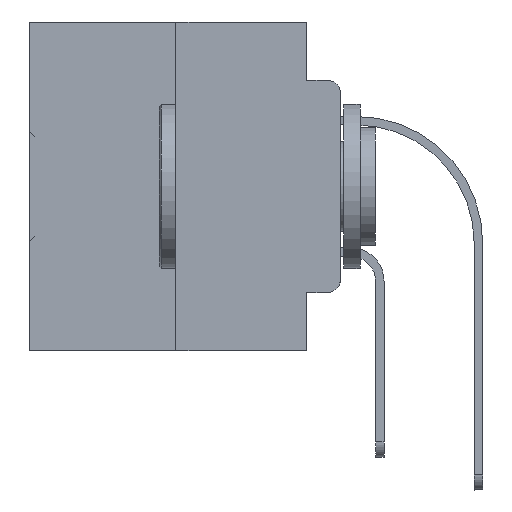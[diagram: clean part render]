
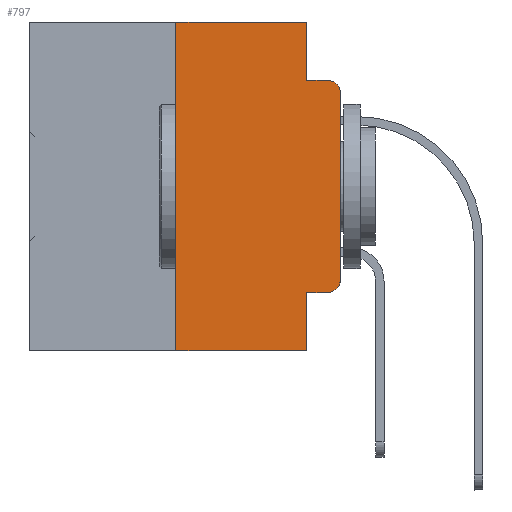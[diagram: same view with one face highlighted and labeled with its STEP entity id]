
A CAD part, left-side view. The second image highlights one B-rep face of the part: STEP entity #797.
In plain terms, the highlighted planar face has unit normal (-1, 0, 0).
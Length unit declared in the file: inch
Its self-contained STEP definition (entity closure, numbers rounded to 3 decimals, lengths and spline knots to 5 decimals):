
#170 = ORIENTED_EDGE ( 'NONE', *, *, #8537, .T. ) ;
#797 = ADVANCED_FACE ( 'NONE', ( #30992 ), #1287, .F. ) ;
#883 = CARTESIAN_POINT ( 'NONE',  ( 0., 0.473, 0. ) ) ;
#1096 = ORIENTED_EDGE ( 'NONE', *, *, #7318, .F. ) ;
#1287 = PLANE ( 'NONE',  #10939 ) ;
#1345 = VERTEX_POINT ( 'NONE', #14039 ) ;
#3352 = CARTESIAN_POINT ( 'NONE',  ( 0., 0.473, -0.5 ) ) ;
#3645 = LINE ( 'NONE', #18437, #16401 ) ;
#3656 = CARTESIAN_POINT ( 'NONE',  ( 0., 0.051, -0.0885 ) ) ;
#4393 = DIRECTION ( 'NONE',  ( 1., 0., 0. ) ) ;
#6863 = CARTESIAN_POINT ( 'NONE',  ( 0., 0., -0.1085 ) ) ;
#6879 = ORIENTED_EDGE ( 'NONE', *, *, #21582, .T. ) ;
#7318 = EDGE_CURVE ( 'NONE', #8456, #8293, #36587, .T. ) ;
#8228 = VECTOR ( 'NONE', #30574, 39.37008 ) ;
#8293 = VERTEX_POINT ( 'NONE', #17442 ) ;
#8456 = VERTEX_POINT ( 'NONE', #23482 ) ;
#8537 = EDGE_CURVE ( 'NONE', #38240, #11302, #30975, .T. ) ;
#8684 = EDGE_CURVE ( 'NONE', #8293, #34382, #36230, .T. ) ;
#8834 = ORIENTED_EDGE ( 'NONE', *, *, #22237, .F. ) ;
#8986 = CARTESIAN_POINT ( 'NONE',  ( 0., 0.02, -0.1085 ) ) ;
#9267 = EDGE_CURVE ( 'NONE', #34382, #1345, #3645, .T. ) ;
#9439 = ORIENTED_EDGE ( 'NONE', *, *, #9267, .F. ) ;
#9651 = CARTESIAN_POINT ( 'NONE',  ( 0., 0.051, 0. ) ) ;
#9960 = VERTEX_POINT ( 'NONE', #31731 ) ;
#10237 = DIRECTION ( 'NONE',  ( 0., 0., -1. ) ) ;
#10436 = AXIS2_PLACEMENT_3D ( 'NONE', #34102, #12779, #10237 ) ;
#10939 = AXIS2_PLACEMENT_3D ( 'NONE', #31196, #4393, #28299 ) ;
#11302 = VERTEX_POINT ( 'NONE', #36538 ) ;
#11423 = DIRECTION ( 'NONE',  ( 0., 0., 1. ) ) ;
#12779 = DIRECTION ( 'NONE',  ( -1., 0., 0. ) ) ;
#12907 = CIRCLE ( 'NONE', #10436, 0.02 ) ;
#13124 = CARTESIAN_POINT ( 'NONE',  ( 0., 0., 0. ) ) ;
#13659 = ORIENTED_EDGE ( 'NONE', *, *, #18242, .T. ) ;
#13963 = CARTESIAN_POINT ( 'NONE',  ( 0., 0.25, 0. ) ) ;
#14039 = CARTESIAN_POINT ( 'NONE',  ( 0., 0.02, -0.0885 ) ) ;
#15121 = VECTOR ( 'NONE', #21505, 39.37008 ) ;
#15213 = DIRECTION ( 'NONE',  ( -1., 0., 0. ) ) ;
#16401 = VECTOR ( 'NONE', #27344, 39.37008 ) ;
#16429 = ORIENTED_EDGE ( 'NONE', *, *, #33892, .F. ) ;
#16442 = LINE ( 'NONE', #13124, #35106 ) ;
#17060 = LINE ( 'NONE', #13963, #34135 ) ;
#17442 = CARTESIAN_POINT ( 'NONE',  ( 0., 0.051, 0. ) ) ;
#18242 = EDGE_CURVE ( 'NONE', #11302, #36356, #12907, .T. ) ;
#18368 = ORIENTED_EDGE ( 'NONE', *, *, #29549, .T. ) ;
#18437 = CARTESIAN_POINT ( 'NONE',  ( 0., 0.051, -0.0885 ) ) ;
#18628 = VERTEX_POINT ( 'NONE', #6863 ) ;
#18698 = LINE ( 'NONE', #3352, #23615 ) ;
#21505 = DIRECTION ( 'NONE',  ( 0., 0., -1. ) ) ;
#21578 = EDGE_CURVE ( 'NONE', #9960, #29554, #18698, .T. ) ;
#21582 = EDGE_CURVE ( 'NONE', #18628, #1345, #22959, .T. ) ;
#22237 = EDGE_CURVE ( 'NONE', #9960, #8456, #17060, .T. ) ;
#22653 = CARTESIAN_POINT ( 'NONE',  ( 0., 0.051, -0.5 ) ) ;
#22959 = CIRCLE ( 'NONE', #27899, 0.02 ) ;
#23482 = CARTESIAN_POINT ( 'NONE',  ( 0., 0.25, 0. ) ) ;
#23615 = VECTOR ( 'NONE', #26687, 39.37008 ) ;
#23784 = VECTOR ( 'NONE', #33321, 39.37008 ) ;
#25923 = CARTESIAN_POINT ( 'NONE',  ( 0., 0.051, -0.4115 ) ) ;
#26552 = CARTESIAN_POINT ( 'NONE',  ( 0., 0.051, 0. ) ) ;
#26687 = DIRECTION ( 'NONE',  ( 0., -1., 0. ) ) ;
#27063 = DIRECTION ( 'NONE',  ( 0., 0., -1. ) ) ;
#27344 = DIRECTION ( 'NONE',  ( 0., -1., 0. ) ) ;
#27899 = AXIS2_PLACEMENT_3D ( 'NONE', #8986, #15213, #27063 ) ;
#28273 = DIRECTION ( 'NONE',  ( 0., 0., 1. ) ) ;
#28299 = DIRECTION ( 'NONE',  ( 0., 0., -1. ) ) ;
#29549 = EDGE_CURVE ( 'NONE', #36356, #18628, #16442, .T. ) ;
#29554 = VERTEX_POINT ( 'NONE', #22653 ) ;
#30574 = DIRECTION ( 'NONE',  ( 0., -1., 0. ) ) ;
#30586 = CARTESIAN_POINT ( 'NONE',  ( 0., 0.051, -0.4115 ) ) ;
#30674 = ORIENTED_EDGE ( 'NONE', *, *, #8684, .F. ) ;
#30975 = LINE ( 'NONE', #30586, #23784 ) ;
#30992 = FACE_OUTER_BOUND ( 'NONE', #31479, .T. ) ;
#31172 = VECTOR ( 'NONE', #32154, 39.37008 ) ;
#31196 = CARTESIAN_POINT ( 'NONE',  ( 0., 0.473, 0. ) ) ;
#31479 = EDGE_LOOP ( 'NONE', ( #18368, #6879, #9439, #30674, #1096, #8834, #33101, #16429, #170, #13659 ) ) ;
#31731 = CARTESIAN_POINT ( 'NONE',  ( 0., 0.25, -0.5 ) ) ;
#31765 = LINE ( 'NONE', #26552, #31172 ) ;
#32145 = CARTESIAN_POINT ( 'NONE',  ( 0., 0., -0.3915 ) ) ;
#32154 = DIRECTION ( 'NONE',  ( 0., 0., -1. ) ) ;
#33101 = ORIENTED_EDGE ( 'NONE', *, *, #21578, .T. ) ;
#33321 = DIRECTION ( 'NONE',  ( 0., -1., 0. ) ) ;
#33892 = EDGE_CURVE ( 'NONE', #38240, #29554, #31765, .T. ) ;
#34102 = CARTESIAN_POINT ( 'NONE',  ( 0., 0.02, -0.3915 ) ) ;
#34135 = VECTOR ( 'NONE', #11423, 39.37008 ) ;
#34382 = VERTEX_POINT ( 'NONE', #3656 ) ;
#35106 = VECTOR ( 'NONE', #28273, 39.37008 ) ;
#36230 = LINE ( 'NONE', #9651, #15121 ) ;
#36356 = VERTEX_POINT ( 'NONE', #32145 ) ;
#36538 = CARTESIAN_POINT ( 'NONE',  ( 0., 0.02, -0.4115 ) ) ;
#36587 = LINE ( 'NONE', #883, #8228 ) ;
#38240 = VERTEX_POINT ( 'NONE', #25923 ) ;
